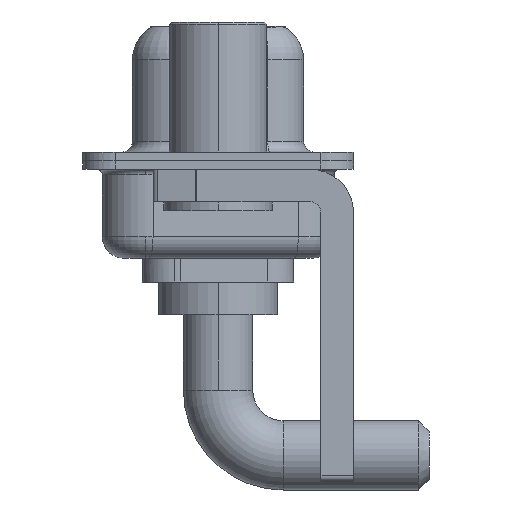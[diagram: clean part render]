
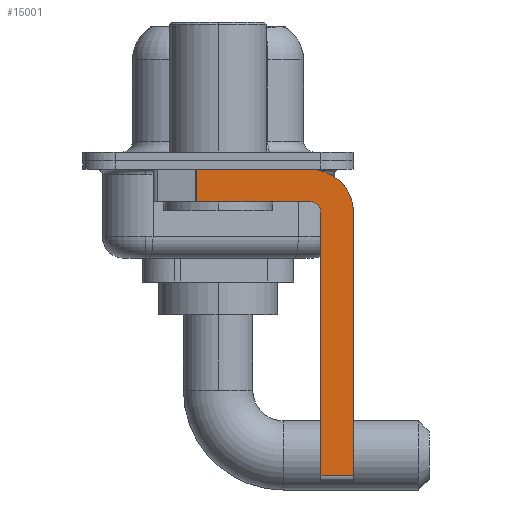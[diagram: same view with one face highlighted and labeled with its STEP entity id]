
A CAD part, left-side view. The second image highlights one B-rep face of the part: STEP entity #15001.
In plain terms, the highlighted planar face has unit normal (-1, 0, 0).
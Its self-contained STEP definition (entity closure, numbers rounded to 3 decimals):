
#19 = CARTESIAN_POINT ( 'NONE',  ( -2.9, -4.25, -1.9 ) ) ;
#58 = CARTESIAN_POINT ( 'NONE',  ( -2.9, -6.25, -2.4 ) ) ;
#945 = VECTOR ( 'NONE', #9305, 1000. ) ;
#1157 = CARTESIAN_POINT ( 'NONE',  ( -2.9, -4.75, -14.55 ) ) ;
#1299 = CARTESIAN_POINT ( 'NONE',  ( -2.9, -4.25, -1.9 ) ) ;
#1323 = EDGE_CURVE ( 'NONE', #15197, #8023, #6129, .T. ) ;
#1496 = PLANE ( 'NONE',  #13316 ) ;
#1507 = VECTOR ( 'NONE', #2891, 1000. ) ;
#1517 = EDGE_CURVE ( 'NONE', #3184, #3815, #5091, .T. ) ;
#1616 = CARTESIAN_POINT ( 'NONE',  ( -2.9, 0.978, -0.4 ) ) ;
#1736 = AXIS2_PLACEMENT_3D ( 'NONE', #14735, #6157, #5038 ) ;
#2059 = ORIENTED_EDGE ( 'NONE', *, *, #1323, .T. ) ;
#2116 = VERTEX_POINT ( 'NONE', #9131 ) ;
#2141 = EDGE_LOOP ( 'NONE', ( #2955, #6678, #3500, #9584, #8861, #2059, #4446, #5813 ) ) ;
#2467 = DIRECTION ( 'NONE',  ( 0., 0., -1. ) ) ;
#2560 = LINE ( 'NONE', #4014, #1507 ) ;
#2891 = DIRECTION ( 'NONE',  ( 0., 0., 1. ) ) ;
#2955 = ORIENTED_EDGE ( 'NONE', *, *, #7227, .F. ) ;
#3052 = FACE_OUTER_BOUND ( 'NONE', #2141, .T. ) ;
#3184 = VERTEX_POINT ( 'NONE', #19 ) ;
#3364 = VECTOR ( 'NONE', #4774, 1000. ) ;
#3500 = ORIENTED_EDGE ( 'NONE', *, *, #1517, .F. ) ;
#3577 = VECTOR ( 'NONE', #4984, 1000. ) ;
#3604 = LINE ( 'NONE', #3690, #8746 ) ;
#3690 = CARTESIAN_POINT ( 'NONE',  ( -2.9, 0.978, -1.9 ) ) ;
#3696 = CARTESIAN_POINT ( 'NONE',  ( -2.9, -6.25, -2.4 ) ) ;
#3815 = VERTEX_POINT ( 'NONE', #11533 ) ;
#3852 = DIRECTION ( 'NONE',  ( 0., 0., -1. ) ) ;
#4014 = CARTESIAN_POINT ( 'NONE',  ( -2.9, -4.75, -14.8 ) ) ;
#4446 = ORIENTED_EDGE ( 'NONE', *, *, #9068, .F. ) ;
#4774 = DIRECTION ( 'NONE',  ( 0., -1., 0. ) ) ;
#4982 = EDGE_CURVE ( 'NONE', #12988, #3815, #3604, .T. ) ;
#4984 = DIRECTION ( 'NONE',  ( 0., 0., -1. ) ) ;
#5038 = DIRECTION ( 'NONE',  ( 0., 0., 1. ) ) ;
#5082 = CIRCLE ( 'NONE', #1736, 0.5 ) ;
#5091 = LINE ( 'NONE', #1299, #8074 ) ;
#5813 = ORIENTED_EDGE ( 'NONE', *, *, #8974, .F. ) ;
#6129 = LINE ( 'NONE', #10678, #3364 ) ;
#6157 = DIRECTION ( 'NONE',  ( -1., 0., 0. ) ) ;
#6570 = DIRECTION ( 'NONE',  ( 0., 0., -1. ) ) ;
#6644 = CARTESIAN_POINT ( 'NONE',  ( -2.9, -4.25, -2.4 ) ) ;
#6678 = ORIENTED_EDGE ( 'NONE', *, *, #4982, .T. ) ;
#7227 = EDGE_CURVE ( 'NONE', #12988, #15198, #8258, .T. ) ;
#7455 = CARTESIAN_POINT ( 'NONE',  ( -2.9, -4.25, -2.4 ) ) ;
#7647 = DIRECTION ( 'NONE',  ( 0., 1., 0. ) ) ;
#7856 = EDGE_CURVE ( 'NONE', #2116, #3184, #5082, .T. ) ;
#8023 = VERTEX_POINT ( 'NONE', #13635 ) ;
#8074 = VECTOR ( 'NONE', #7647, 1000. ) ;
#8258 = LINE ( 'NONE', #8335, #945 ) ;
#8335 = CARTESIAN_POINT ( 'NONE',  ( -2.9, 3., -0.4 ) ) ;
#8643 = DIRECTION ( 'NONE',  ( 1., 0., 0. ) ) ;
#8746 = VECTOR ( 'NONE', #2467, 1000. ) ;
#8861 = ORIENTED_EDGE ( 'NONE', *, *, #9054, .F. ) ;
#8974 = EDGE_CURVE ( 'NONE', #15198, #14825, #12760, .T. ) ;
#9054 = EDGE_CURVE ( 'NONE', #15197, #2116, #2560, .T. ) ;
#9068 = EDGE_CURVE ( 'NONE', #14825, #8023, #11042, .T. ) ;
#9131 = CARTESIAN_POINT ( 'NONE',  ( -2.9, -4.75, -2.4 ) ) ;
#9305 = DIRECTION ( 'NONE',  ( 0., -1., 0. ) ) ;
#9584 = ORIENTED_EDGE ( 'NONE', *, *, #7856, .F. ) ;
#10678 = CARTESIAN_POINT ( 'NONE',  ( -2.9, -4.25, -14.55 ) ) ;
#10974 = AXIS2_PLACEMENT_3D ( 'NONE', #7455, #8643, #3852 ) ;
#11042 = LINE ( 'NONE', #58, #3577 ) ;
#11514 = DIRECTION ( 'NONE',  ( 1., 0., 0. ) ) ;
#11533 = CARTESIAN_POINT ( 'NONE',  ( -2.9, 0.978, -1.9 ) ) ;
#12143 = CARTESIAN_POINT ( 'NONE',  ( -2.9, -4.25, -0.4 ) ) ;
#12760 = CIRCLE ( 'NONE', #10974, 2. ) ;
#12988 = VERTEX_POINT ( 'NONE', #1616 ) ;
#13316 = AXIS2_PLACEMENT_3D ( 'NONE', #6644, #11514, #6570 ) ;
#13635 = CARTESIAN_POINT ( 'NONE',  ( -2.9, -6.25, -14.55 ) ) ;
#14735 = CARTESIAN_POINT ( 'NONE',  ( -2.9, -4.25, -2.4 ) ) ;
#14825 = VERTEX_POINT ( 'NONE', #3696 ) ;
#15001 = ADVANCED_FACE ( 'NONE', ( #3052 ), #1496, .F. ) ;
#15197 = VERTEX_POINT ( 'NONE', #1157 ) ;
#15198 = VERTEX_POINT ( 'NONE', #12143 ) ;
